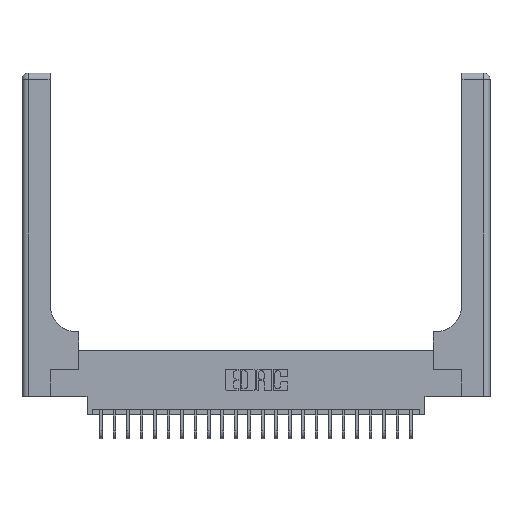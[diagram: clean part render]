
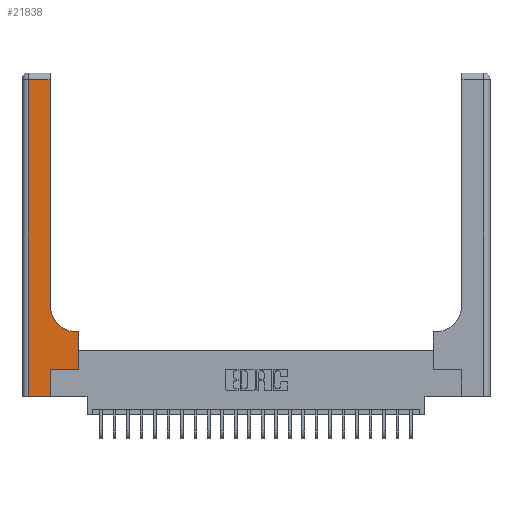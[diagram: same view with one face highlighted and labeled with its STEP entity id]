
A CAD part, top view. The second image highlights one B-rep face of the part: STEP entity #21838.
In plain terms, the highlighted planar face has unit normal (0, 0, 1).
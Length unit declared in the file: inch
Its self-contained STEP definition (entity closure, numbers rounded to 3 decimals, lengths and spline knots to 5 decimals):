
#543 = ORIENTED_EDGE ( 'NONE', *, *, #10918, .T. ) ;
#650 = CARTESIAN_POINT ( 'NONE',  ( 0.26, 0.85, 0.37 ) ) ;
#1440 = CARTESIAN_POINT ( 'NONE',  ( 0.528, 0.6, 0.37 ) ) ;
#1557 = CARTESIAN_POINT ( 'NONE',  ( 0.265, 0., 0.37 ) ) ;
#1624 = VECTOR ( 'NONE', #5820, 39.37008 ) ;
#1797 = CARTESIAN_POINT ( 'NONE',  ( 0.528, 0.25, 0.37 ) ) ;
#1870 = DIRECTION ( 'NONE',  ( -1., 0., 0. ) ) ;
#1964 = ORIENTED_EDGE ( 'NONE', *, *, #16452, .T. ) ;
#2468 = DIRECTION ( 'NONE',  ( 0., -1., 0. ) ) ;
#2868 = VERTEX_POINT ( 'NONE', #650 ) ;
#3779 = VERTEX_POINT ( 'NONE', #1440 ) ;
#4128 = LINE ( 'NONE', #13835, #19648 ) ;
#4176 = VERTEX_POINT ( 'NONE', #22155 ) ;
#4515 = VECTOR ( 'NONE', #7462, 39.37008 ) ;
#4770 = CARTESIAN_POINT ( 'NONE',  ( 0.51, 0.6, 0.37 ) ) ;
#4792 = DIRECTION ( 'NONE',  ( 0., 0., -1. ) ) ;
#4876 = ORIENTED_EDGE ( 'NONE', *, *, #21724, .T. ) ;
#4948 = VECTOR ( 'NONE', #8433, 39.37008 ) ;
#5820 = DIRECTION ( 'NONE',  ( 0., 1., 0. ) ) ;
#6342 = CARTESIAN_POINT ( 'NONE',  ( 0., 2.94, 0.37 ) ) ;
#6814 = ORIENTED_EDGE ( 'NONE', *, *, #17078, .T. ) ;
#6975 = VERTEX_POINT ( 'NONE', #4770 ) ;
#7093 = LINE ( 'NONE', #9401, #22908 ) ;
#7424 = EDGE_CURVE ( 'NONE', #6975, #2868, #22351, .T. ) ;
#7462 = DIRECTION ( 'NONE',  ( 0., 1., 0. ) ) ;
#7875 = DIRECTION ( 'NONE',  ( 0., 1., 0. ) ) ;
#7876 = VECTOR ( 'NONE', #7875, 39.37008 ) ;
#8190 = LINE ( 'NONE', #19639, #16446 ) ;
#8433 = DIRECTION ( 'NONE',  ( -1., 0., 0. ) ) ;
#8472 = ORIENTED_EDGE ( 'NONE', *, *, #24408, .T. ) ;
#9401 = CARTESIAN_POINT ( 'NONE',  ( 0.265, 0.25, 0.37 ) ) ;
#9847 = LINE ( 'NONE', #23352, #1624 ) ;
#10202 = CARTESIAN_POINT ( 'NONE',  ( 0.528, 0.25, 0.37 ) ) ;
#10918 = EDGE_CURVE ( 'NONE', #2868, #20396, #13072, .T. ) ;
#11027 = VERTEX_POINT ( 'NONE', #18017 ) ;
#11500 = ORIENTED_EDGE ( 'NONE', *, *, #21285, .T. ) ;
#13072 = LINE ( 'NONE', #13792, #7876 ) ;
#13269 = AXIS2_PLACEMENT_3D ( 'NONE', #17705, #19474, #1870 ) ;
#13792 = CARTESIAN_POINT ( 'NONE',  ( 0.26, 3., 0.37 ) ) ;
#13835 = CARTESIAN_POINT ( 'NONE',  ( 0., 0., 0.37 ) ) ;
#13884 = LINE ( 'NONE', #6342, #16347 ) ;
#13961 = DIRECTION ( 'NONE',  ( -1., 0., 0. ) ) ;
#14211 = EDGE_CURVE ( 'NONE', #3779, #6975, #17164, .T. ) ;
#14920 = ORIENTED_EDGE ( 'NONE', *, *, #14211, .T. ) ;
#15023 = CARTESIAN_POINT ( 'NONE',  ( 0.265, 0.25, 0.37 ) ) ;
#15211 = VERTEX_POINT ( 'NONE', #1557 ) ;
#15507 = AXIS2_PLACEMENT_3D ( 'NONE', #20441, #4792, #22624 ) ;
#15520 = LINE ( 'NONE', #1797, #4515 ) ;
#16347 = VECTOR ( 'NONE', #13961, 39.37008 ) ;
#16374 = CARTESIAN_POINT ( 'NONE',  ( 0.26, 0.6, 0.37 ) ) ;
#16446 = VECTOR ( 'NONE', #2468, 39.37008 ) ;
#16452 = EDGE_CURVE ( 'NONE', #11027, #15211, #4128, .T. ) ;
#17078 = EDGE_CURVE ( 'NONE', #20396, #4176, #13884, .T. ) ;
#17164 = LINE ( 'NONE', #16374, #4948 ) ;
#17253 = DIRECTION ( 'NONE',  ( 1., 0., 0. ) ) ;
#17705 = CARTESIAN_POINT ( 'NONE',  ( 0., 3., 0.37 ) ) ;
#17726 = DIRECTION ( 'NONE',  ( 1., 0., 0. ) ) ;
#18017 = CARTESIAN_POINT ( 'NONE',  ( 0.06, 0., 0.37 ) ) ;
#18682 = EDGE_CURVE ( 'NONE', #18984, #25169, #7093, .T. ) ;
#18984 = VERTEX_POINT ( 'NONE', #15023 ) ;
#19035 = CARTESIAN_POINT ( 'NONE',  ( 0.26, 2.94, 0.37 ) ) ;
#19474 = DIRECTION ( 'NONE',  ( 0., 0., -1. ) ) ;
#19639 = CARTESIAN_POINT ( 'NONE',  ( 0.06, 3., 0.37 ) ) ;
#19648 = VECTOR ( 'NONE', #17726, 39.37008 ) ;
#20396 = VERTEX_POINT ( 'NONE', #19035 ) ;
#20441 = CARTESIAN_POINT ( 'NONE',  ( 0.51, 0.85, 0.37 ) ) ;
#20620 = FACE_OUTER_BOUND ( 'NONE', #22446, .T. ) ;
#21057 = ORIENTED_EDGE ( 'NONE', *, *, #18682, .T. ) ;
#21285 = EDGE_CURVE ( 'NONE', #4176, #11027, #8190, .T. ) ;
#21575 = PLANE ( 'NONE',  #13269 ) ;
#21724 = EDGE_CURVE ( 'NONE', #25169, #3779, #15520, .T. ) ;
#21838 = ADVANCED_FACE ( 'NONE', ( #20620 ), #21575, .F. ) ;
#22155 = CARTESIAN_POINT ( 'NONE',  ( 0.06, 2.94, 0.37 ) ) ;
#22351 = CIRCLE ( 'NONE', #15507, 0.25 ) ;
#22446 = EDGE_LOOP ( 'NONE', ( #543, #6814, #11500, #1964, #8472, #21057, #4876, #14920, #24898 ) ) ;
#22624 = DIRECTION ( 'NONE',  ( 1., 0., 0. ) ) ;
#22908 = VECTOR ( 'NONE', #17253, 39.37008 ) ;
#23352 = CARTESIAN_POINT ( 'NONE',  ( 0.265, 0., 0.37 ) ) ;
#24408 = EDGE_CURVE ( 'NONE', #15211, #18984, #9847, .T. ) ;
#24898 = ORIENTED_EDGE ( 'NONE', *, *, #7424, .T. ) ;
#25169 = VERTEX_POINT ( 'NONE', #10202 ) ;
